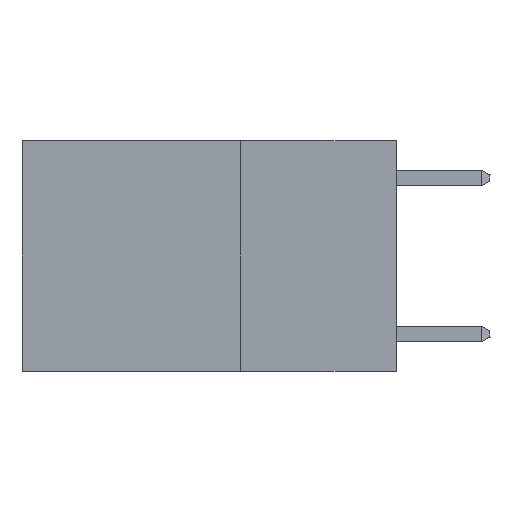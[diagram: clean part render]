
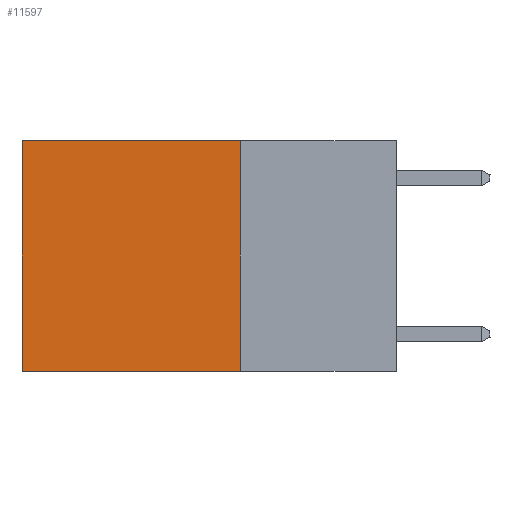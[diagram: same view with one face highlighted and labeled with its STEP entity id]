
A CAD part, left-side view. The second image highlights one B-rep face of the part: STEP entity #11597.
In plain terms, the highlighted planar face has unit normal (-1, 0, 0).
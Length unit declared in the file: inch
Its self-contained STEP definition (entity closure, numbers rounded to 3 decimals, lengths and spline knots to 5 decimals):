
#527 = EDGE_CURVE ( 'NONE', #7715, #7485, #11501, .T. ) ;
#541 = EDGE_CURVE ( 'NONE', #11265, #7485, #1489, .T. ) ;
#639 = VECTOR ( 'NONE', #1740, 39.37008 ) ;
#740 = CARTESIAN_POINT ( 'NONE',  ( 0.2625, 0.25, 0. ) ) ;
#929 = DIRECTION ( 'NONE',  ( 1., 0., 0. ) ) ;
#1229 = EDGE_CURVE ( 'NONE', #3404, #7715, #11113, .T. ) ;
#1489 = LINE ( 'NONE', #11689, #2349 ) ;
#1527 = EDGE_CURVE ( 'NONE', #3404, #11265, #8234, .T. ) ;
#1740 = DIRECTION ( 'NONE',  ( 0., 0., -1. ) ) ;
#2349 = VECTOR ( 'NONE', #7959, 39.37008 ) ;
#3404 = VERTEX_POINT ( 'NONE', #740 ) ;
#4681 = DIRECTION ( 'NONE',  ( 0., 1., 0. ) ) ;
#5296 = VECTOR ( 'NONE', #4681, 39.37008 ) ;
#5720 = CARTESIAN_POINT ( 'NONE',  ( 0.2625, 0.25, 0. ) ) ;
#5984 = DIRECTION ( 'NONE',  ( 0., 0., -1. ) ) ;
#6369 = ORIENTED_EDGE ( 'NONE', *, *, #527, .T. ) ;
#6395 = FACE_OUTER_BOUND ( 'NONE', #8593, .T. ) ;
#6416 = AXIS2_PLACEMENT_3D ( 'NONE', #10149, #929, #8264 ) ;
#7485 = VERTEX_POINT ( 'NONE', #10060 ) ;
#7715 = VERTEX_POINT ( 'NONE', #8679 ) ;
#7903 = CARTESIAN_POINT ( 'NONE',  ( 0.2625, 0.6, 0. ) ) ;
#7959 = DIRECTION ( 'NONE',  ( 0., 1., 0. ) ) ;
#8234 = LINE ( 'NONE', #9206, #639 ) ;
#8264 = DIRECTION ( 'NONE',  ( 0., 0., -1. ) ) ;
#8432 = PLANE ( 'NONE',  #6416 ) ;
#8593 = EDGE_LOOP ( 'NONE', ( #6369, #9492, #9328, #10774 ) ) ;
#8679 = CARTESIAN_POINT ( 'NONE',  ( 0.2625, 0.6, 0. ) ) ;
#9206 = CARTESIAN_POINT ( 'NONE',  ( 0.2625, 0.25, 0. ) ) ;
#9328 = ORIENTED_EDGE ( 'NONE', *, *, #1527, .F. ) ;
#9492 = ORIENTED_EDGE ( 'NONE', *, *, #541, .F. ) ;
#10060 = CARTESIAN_POINT ( 'NONE',  ( 0.2625, 0.6, -0.37 ) ) ;
#10149 = CARTESIAN_POINT ( 'NONE',  ( 0.2625, 0.25, 0. ) ) ;
#10774 = ORIENTED_EDGE ( 'NONE', *, *, #1229, .T. ) ;
#11066 = CARTESIAN_POINT ( 'NONE',  ( 0.2625, 0.25, -0.37 ) ) ;
#11113 = LINE ( 'NONE', #5720, #5296 ) ;
#11265 = VERTEX_POINT ( 'NONE', #11066 ) ;
#11310 = VECTOR ( 'NONE', #5984, 39.37008 ) ;
#11501 = LINE ( 'NONE', #7903, #11310 ) ;
#11597 = ADVANCED_FACE ( 'NONE', ( #6395 ), #8432, .F. ) ;
#11689 = CARTESIAN_POINT ( 'NONE',  ( 0.2625, 0.25, -0.37 ) ) ;
